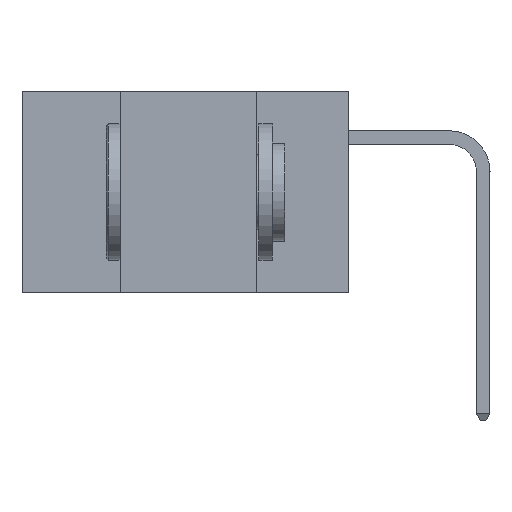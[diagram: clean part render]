
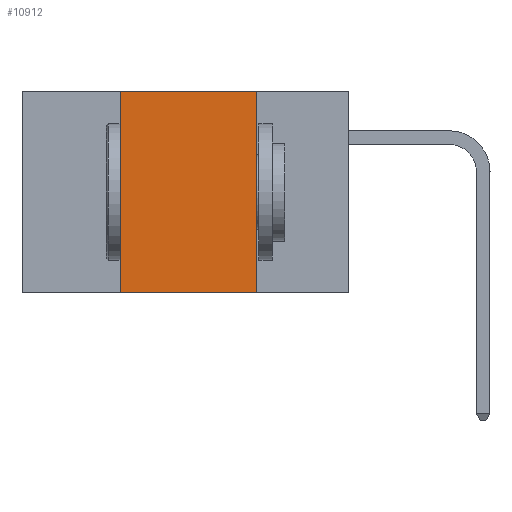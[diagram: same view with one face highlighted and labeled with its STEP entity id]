
A CAD part, left-side view. The second image highlights one B-rep face of the part: STEP entity #10912.
In plain terms, the highlighted planar face has unit normal (-1, 0, 0).
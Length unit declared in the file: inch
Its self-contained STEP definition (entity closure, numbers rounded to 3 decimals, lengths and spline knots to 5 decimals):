
#278 = VERTEX_POINT ( 'NONE', #16354 ) ;
#464 = EDGE_CURVE ( 'NONE', #13293, #34336, #22272, .T. ) ;
#931 = EDGE_LOOP ( 'NONE', ( #23514, #18608, #20371, #31486 ) ) ;
#8264 = EDGE_CURVE ( 'NONE', #13293, #28265, #12139, .T. ) ;
#8818 = DIRECTION ( 'NONE',  ( 0., -1., 0. ) ) ;
#9004 = PLANE ( 'NONE',  #29836 ) ;
#9842 = CARTESIAN_POINT ( 'NONE',  ( 0., 0.17, 0. ) ) ;
#10619 = CARTESIAN_POINT ( 'NONE',  ( 0., 0.42, 0. ) ) ;
#10912 = ADVANCED_FACE ( 'NONE', ( #22191 ), #9004, .F. ) ;
#11751 = CARTESIAN_POINT ( 'NONE',  ( 0., 0.6, -0.37 ) ) ;
#12139 = LINE ( 'NONE', #13490, #17935 ) ;
#13293 = VERTEX_POINT ( 'NONE', #14148 ) ;
#13490 = CARTESIAN_POINT ( 'NONE',  ( 0., 0.42, 0. ) ) ;
#13650 = LINE ( 'NONE', #34753, #34470 ) ;
#14148 = CARTESIAN_POINT ( 'NONE',  ( 0., 0.42, -0.37 ) ) ;
#14799 = DIRECTION ( 'NONE',  ( 0., 0., -1. ) ) ;
#14936 = DIRECTION ( 'NONE',  ( 0., -1., 0. ) ) ;
#16283 = LINE ( 'NONE', #9842, #31080 ) ;
#16354 = CARTESIAN_POINT ( 'NONE',  ( 0., 0.17, 0. ) ) ;
#16454 = CARTESIAN_POINT ( 'NONE',  ( 0., 0.17, -0.37 ) ) ;
#17889 = EDGE_CURVE ( 'NONE', #278, #34336, #16283, .T. ) ;
#17935 = VECTOR ( 'NONE', #21952, 39.37008 ) ;
#18608 = ORIENTED_EDGE ( 'NONE', *, *, #35223, .F. ) ;
#20371 = ORIENTED_EDGE ( 'NONE', *, *, #8264, .F. ) ;
#21952 = DIRECTION ( 'NONE',  ( 0., 0., 1. ) ) ;
#22191 = FACE_OUTER_BOUND ( 'NONE', #931, .T. ) ;
#22272 = LINE ( 'NONE', #11751, #36395 ) ;
#23514 = ORIENTED_EDGE ( 'NONE', *, *, #17889, .F. ) ;
#28265 = VERTEX_POINT ( 'NONE', #10619 ) ;
#28982 = CARTESIAN_POINT ( 'NONE',  ( 0., 0.6, 0. ) ) ;
#29836 = AXIS2_PLACEMENT_3D ( 'NONE', #28982, #31810, #14799 ) ;
#31080 = VECTOR ( 'NONE', #32608, 39.37008 ) ;
#31486 = ORIENTED_EDGE ( 'NONE', *, *, #464, .T. ) ;
#31810 = DIRECTION ( 'NONE',  ( 1., 0., 0. ) ) ;
#32608 = DIRECTION ( 'NONE',  ( 0., 0., -1. ) ) ;
#34336 = VERTEX_POINT ( 'NONE', #16454 ) ;
#34470 = VECTOR ( 'NONE', #14936, 39.37008 ) ;
#34753 = CARTESIAN_POINT ( 'NONE',  ( 0., 0.6, 0. ) ) ;
#35223 = EDGE_CURVE ( 'NONE', #28265, #278, #13650, .T. ) ;
#36395 = VECTOR ( 'NONE', #8818, 39.37008 ) ;
